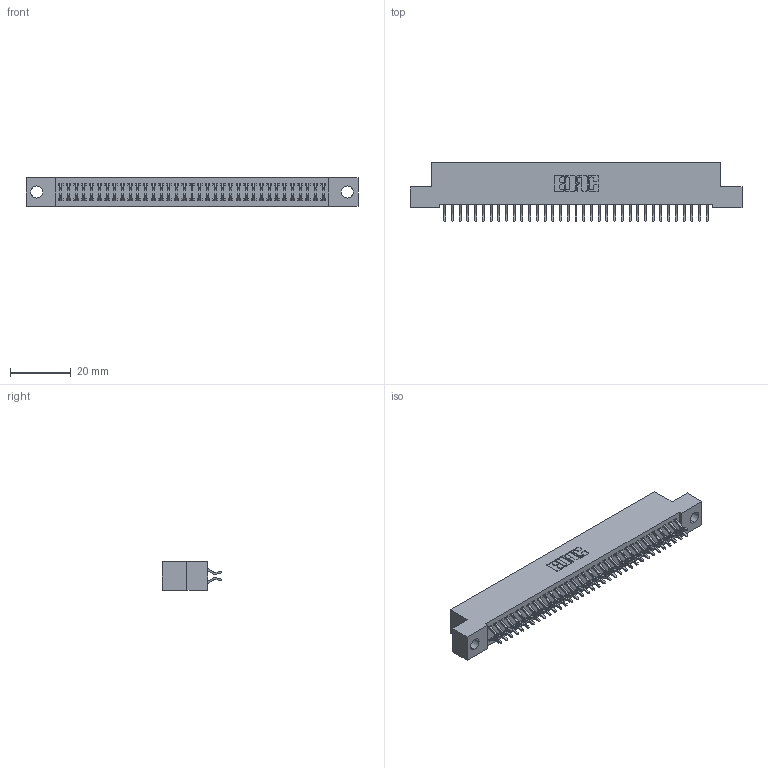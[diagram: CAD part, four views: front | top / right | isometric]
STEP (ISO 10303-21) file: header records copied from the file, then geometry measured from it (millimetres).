
FILE_DESCRIPTION (( 'STEP AP203' ), '1' );
FILE_NAME ('342-070-556-204.STEP', '2019-10-03T16:13:49', ( '' ), ( '' ), 'SwSTEP 2.0', 'SolidWorks 2016', '' );
FILE_SCHEMA (( 'CONFIG_CONTROL_DESIGN' ));
Length unit declared in the file: inch
Products named in the file (3): 342 Part_.156 TH; 345-292-001_556 Tail; 342-070-556-204
Assembly tree (71 placements, depth 2):
  342-070-556-204
    342 Part_.156 TH
    345-292-001_556 Tail  x70
Bounding box: 109.22 x 19.58 x 9.4 mm (x, y, z)
Volume: 9691.5 mm3; surface area: 15359.1 mm2
Topology: 71 solids, 71 shells, 4170 faces, 12409 edges, 8178 vertices
Faces by surface type: plane 2866, cylinder 1304
Entity records: 23513 total; most frequent: CARTESIAN_POINT 3918, ORIENTED_EDGE 3842, DIRECTION 3349, EDGE_CURVE 1921, VECTOR 1785, LINE 1785, VERTEX_POINT 1278, AXIS2_PLACEMENT_3D 782
